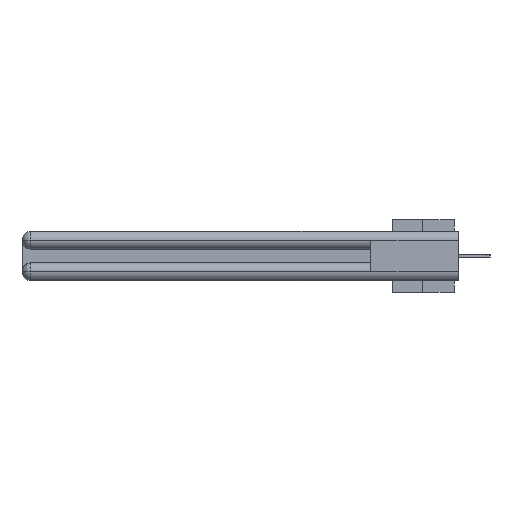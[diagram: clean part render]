
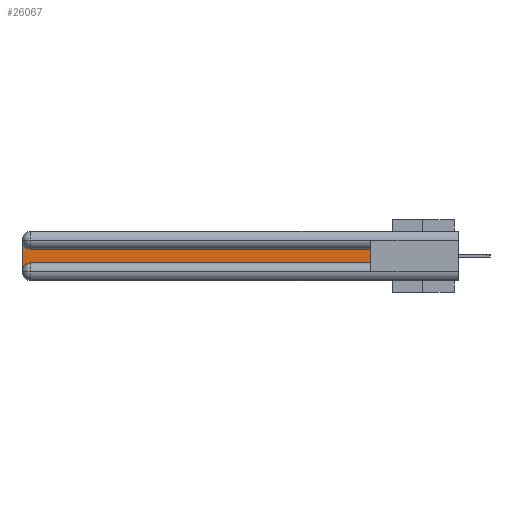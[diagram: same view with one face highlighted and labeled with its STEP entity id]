
A CAD part, left-side view. The second image highlights one B-rep face of the part: STEP entity #26067.
In plain terms, the highlighted planar face has unit normal (-1, 0, 0).
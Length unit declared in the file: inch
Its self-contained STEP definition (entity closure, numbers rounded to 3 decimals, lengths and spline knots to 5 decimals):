
#175 = DIRECTION ( 'NONE',  ( 1., 0., 0. ) ) ;
#355 = AXIS2_PLACEMENT_3D ( 'NONE', #12897, #175, #22363 ) ;
#2114 = ORIENTED_EDGE ( 'NONE', *, *, #37088, .T. ) ;
#2180 = DIRECTION ( 'NONE',  ( 0., 1., 0. ) ) ;
#2277 = DIRECTION ( 'NONE',  ( 1., 0., 0. ) ) ;
#2290 = EDGE_CURVE ( 'NONE', #11792, #31310, #8495, .T. ) ;
#5917 = CARTESIAN_POINT ( 'NONE',  ( 0.075, 2.94, -0.2175 ) ) ;
#6093 = VERTEX_POINT ( 'NONE', #39841 ) ;
#6319 = CARTESIAN_POINT ( 'NONE',  ( 0.075, 3., -0.0625 ) ) ;
#7737 = LINE ( 'NONE', #38011, #40189 ) ;
#8495 = LINE ( 'NONE', #18039, #32567 ) ;
#11071 = DIRECTION ( 'NONE',  ( 1., 0., 0. ) ) ;
#11792 = VERTEX_POINT ( 'NONE', #40797 ) ;
#11850 = EDGE_CURVE ( 'NONE', #17108, #13592, #7737, .T. ) ;
#12241 = EDGE_LOOP ( 'NONE', ( #20009, #26878, #2114, #37910, #37487, #16714 ) ) ;
#12897 = CARTESIAN_POINT ( 'NONE',  ( 0.075, 3., -0.1225 ) ) ;
#13592 = VERTEX_POINT ( 'NONE', #30837 ) ;
#15324 = FACE_OUTER_BOUND ( 'NONE', #12241, .T. ) ;
#15531 = DIRECTION ( 'NONE',  ( 0., 0., 1. ) ) ;
#16270 = CARTESIAN_POINT ( 'NONE',  ( 0.075, 3., -0.2175 ) ) ;
#16714 = ORIENTED_EDGE ( 'NONE', *, *, #34493, .T. ) ;
#17108 = VERTEX_POINT ( 'NONE', #5917 ) ;
#18039 = CARTESIAN_POINT ( 'NONE',  ( 0.075, 0.6, -0.1225 ) ) ;
#18930 = VECTOR ( 'NONE', #28900, 39.37008 ) ;
#19162 = LINE ( 'NONE', #31160, #25564 ) ;
#19203 = DIRECTION ( 'NONE',  ( 0., -1., 0. ) ) ;
#20009 = ORIENTED_EDGE ( 'NONE', *, *, #2290, .T. ) ;
#21272 = CARTESIAN_POINT ( 'NONE',  ( 0.075, 2.94, -0.2775 ) ) ;
#22291 = VERTEX_POINT ( 'NONE', #6319 ) ;
#22363 = DIRECTION ( 'NONE',  ( 0., 0., -1. ) ) ;
#24442 = DIRECTION ( 'NONE',  ( 0., 0., -1. ) ) ;
#25564 = VECTOR ( 'NONE', #15531, 39.37008 ) ;
#25666 = CIRCLE ( 'NONE', #38104, 0.06 ) ;
#26067 = ADVANCED_FACE ( 'NONE', ( #15324 ), #37889, .F. ) ;
#26878 = ORIENTED_EDGE ( 'NONE', *, *, #27540, .T. ) ;
#27321 = LINE ( 'NONE', #16270, #18930 ) ;
#27540 = EDGE_CURVE ( 'NONE', #31310, #22291, #33965, .T. ) ;
#28254 = CARTESIAN_POINT ( 'NONE',  ( 0.075, 2.94, -0.1225 ) ) ;
#28900 = DIRECTION ( 'NONE',  ( 0., 0., -1. ) ) ;
#29895 = CARTESIAN_POINT ( 'NONE',  ( 0.075, 2.94, -0.0625 ) ) ;
#30837 = CARTESIAN_POINT ( 'NONE',  ( 0.075, 0.6, -0.2175 ) ) ;
#31160 = CARTESIAN_POINT ( 'NONE',  ( 0.075, 0.6, -0.2175 ) ) ;
#31310 = VERTEX_POINT ( 'NONE', #28254 ) ;
#32567 = VECTOR ( 'NONE', #2180, 39.37008 ) ;
#32571 = EDGE_CURVE ( 'NONE', #6093, #17108, #25666, .T. ) ;
#33003 = DIRECTION ( 'NONE',  ( 0., 0., -1. ) ) ;
#33965 = CIRCLE ( 'NONE', #39556, 0.06 ) ;
#34493 = EDGE_CURVE ( 'NONE', #13592, #11792, #19162, .T. ) ;
#37088 = EDGE_CURVE ( 'NONE', #22291, #6093, #27321, .T. ) ;
#37487 = ORIENTED_EDGE ( 'NONE', *, *, #11850, .T. ) ;
#37889 = PLANE ( 'NONE',  #355 ) ;
#37910 = ORIENTED_EDGE ( 'NONE', *, *, #32571, .T. ) ;
#38011 = CARTESIAN_POINT ( 'NONE',  ( 0.075, 0.6, -0.2175 ) ) ;
#38104 = AXIS2_PLACEMENT_3D ( 'NONE', #21272, #2277, #24442 ) ;
#39556 = AXIS2_PLACEMENT_3D ( 'NONE', #29895, #11071, #33003 ) ;
#39841 = CARTESIAN_POINT ( 'NONE',  ( 0.075, 3., -0.2775 ) ) ;
#40189 = VECTOR ( 'NONE', #19203, 39.37008 ) ;
#40797 = CARTESIAN_POINT ( 'NONE',  ( 0.075, 0.6, -0.1225 ) ) ;
